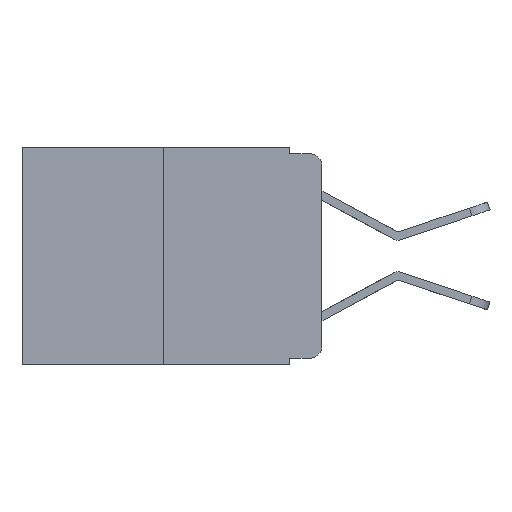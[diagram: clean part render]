
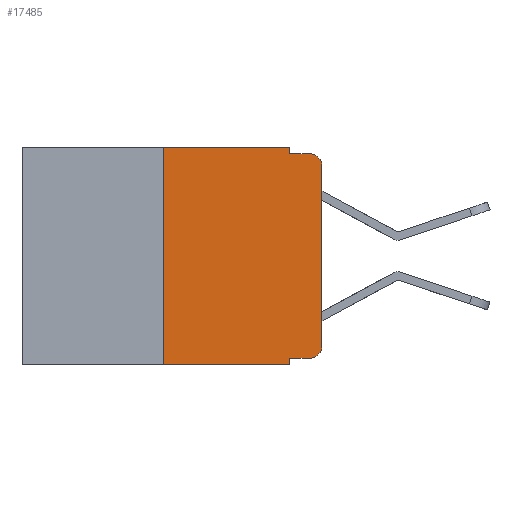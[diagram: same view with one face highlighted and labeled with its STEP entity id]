
A CAD part, left-side view. The second image highlights one B-rep face of the part: STEP entity #17485.
In plain terms, the highlighted planar face has unit normal (-1, 0, 0).
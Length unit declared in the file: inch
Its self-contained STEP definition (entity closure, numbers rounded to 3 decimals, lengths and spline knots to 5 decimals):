
#33 = CARTESIAN_POINT ( 'NONE',  ( 0., 0., -0.03 ) ) ;
#258 = CARTESIAN_POINT ( 'NONE',  ( 0., 0.25, 0. ) ) ;
#469 = LINE ( 'NONE', #2972, #22133 ) ;
#549 = VERTEX_POINT ( 'NONE', #8076 ) ;
#557 = DIRECTION ( 'NONE',  ( 0., 0., -1. ) ) ;
#564 = CARTESIAN_POINT ( 'NONE',  ( 0., 0.051, -0.343 ) ) ;
#1714 = CARTESIAN_POINT ( 'NONE',  ( 0., 0.051, -0.01 ) ) ;
#1905 = VECTOR ( 'NONE', #4295, 39.37008 ) ;
#1937 = AXIS2_PLACEMENT_3D ( 'NONE', #16256, #14419, #10748 ) ;
#1993 = VECTOR ( 'NONE', #10493, 39.37008 ) ;
#2056 = ORIENTED_EDGE ( 'NONE', *, *, #19899, .T. ) ;
#2554 = AXIS2_PLACEMENT_3D ( 'NONE', #11910, #4063, #8116 ) ;
#2972 = CARTESIAN_POINT ( 'NONE',  ( 0., 0.051, -0.333 ) ) ;
#3276 = ORIENTED_EDGE ( 'NONE', *, *, #23657, .T. ) ;
#3572 = CIRCLE ( 'NONE', #2554, 0.02 ) ;
#3613 = VERTEX_POINT ( 'NONE', #564 ) ;
#3642 = DIRECTION ( 'NONE',  ( 0., -1., 0. ) ) ;
#3661 = VERTEX_POINT ( 'NONE', #4584 ) ;
#3707 = LINE ( 'NONE', #8032, #1905 ) ;
#3794 = DIRECTION ( 'NONE',  ( 0., -1., 0. ) ) ;
#4063 = DIRECTION ( 'NONE',  ( -1., 0., 0. ) ) ;
#4295 = DIRECTION ( 'NONE',  ( 0., 0., 1. ) ) ;
#4326 = VERTEX_POINT ( 'NONE', #21395 ) ;
#4584 = CARTESIAN_POINT ( 'NONE',  ( 0., 0.25, -0.343 ) ) ;
#4634 = DIRECTION ( 'NONE',  ( 0., -1., 0. ) ) ;
#4813 = EDGE_CURVE ( 'NONE', #3661, #18534, #3707, .T. ) ;
#5150 = EDGE_CURVE ( 'NONE', #18534, #549, #18207, .T. ) ;
#6787 = CARTESIAN_POINT ( 'NONE',  ( 0., 0.051, 0. ) ) ;
#7406 = VERTEX_POINT ( 'NONE', #22381 ) ;
#7524 = VERTEX_POINT ( 'NONE', #33 ) ;
#8032 = CARTESIAN_POINT ( 'NONE',  ( 0., 0.25, 0. ) ) ;
#8076 = CARTESIAN_POINT ( 'NONE',  ( 0., 0.051, 0. ) ) ;
#8116 = DIRECTION ( 'NONE',  ( 0., 0., -1. ) ) ;
#8274 = EDGE_CURVE ( 'NONE', #8920, #7406, #10379, .T. ) ;
#8920 = VERTEX_POINT ( 'NONE', #23215 ) ;
#9047 = VECTOR ( 'NONE', #14927, 39.37008 ) ;
#9711 = LINE ( 'NONE', #6787, #18607 ) ;
#9781 = ORIENTED_EDGE ( 'NONE', *, *, #4813, .F. ) ;
#9878 = FACE_OUTER_BOUND ( 'NONE', #10364, .T. ) ;
#10024 = PLANE ( 'NONE',  #17247 ) ;
#10364 = EDGE_LOOP ( 'NONE', ( #14322, #15340, #22696, #15757, #14971, #9781, #19636, #17061, #2056, #3276 ) ) ;
#10379 = LINE ( 'NONE', #1714, #12759 ) ;
#10493 = DIRECTION ( 'NONE',  ( 0., 0., -1. ) ) ;
#10511 = DIRECTION ( 'NONE',  ( 0., 0., 1. ) ) ;
#10748 = DIRECTION ( 'NONE',  ( 0., 0., -1. ) ) ;
#11910 = CARTESIAN_POINT ( 'NONE',  ( 0., 0.02, -0.313 ) ) ;
#11927 = DIRECTION ( 'NONE',  ( 1., 0., 0. ) ) ;
#11982 = LINE ( 'NONE', #18602, #9047 ) ;
#12033 = EDGE_CURVE ( 'NONE', #7524, #7406, #23340, .T. ) ;
#12048 = EDGE_CURVE ( 'NONE', #549, #8920, #9711, .T. ) ;
#12759 = VECTOR ( 'NONE', #3642, 39.37008 ) ;
#13300 = VECTOR ( 'NONE', #10511, 39.37008 ) ;
#14263 = CARTESIAN_POINT ( 'NONE',  ( 0., 0.051, 0. ) ) ;
#14322 = ORIENTED_EDGE ( 'NONE', *, *, #23898, .T. ) ;
#14419 = DIRECTION ( 'NONE',  ( -1., 0., 0. ) ) ;
#14667 = DIRECTION ( 'NONE',  ( 0., 0., -1. ) ) ;
#14927 = DIRECTION ( 'NONE',  ( 0., -1., 0. ) ) ;
#14971 = ORIENTED_EDGE ( 'NONE', *, *, #5150, .F. ) ;
#15340 = ORIENTED_EDGE ( 'NONE', *, *, #12033, .T. ) ;
#15757 = ORIENTED_EDGE ( 'NONE', *, *, #12048, .F. ) ;
#16256 = CARTESIAN_POINT ( 'NONE',  ( 0., 0.02, -0.03 ) ) ;
#16284 = CARTESIAN_POINT ( 'NONE',  ( 0., 0., 0. ) ) ;
#16667 = EDGE_CURVE ( 'NONE', #3661, #3613, #11982, .T. ) ;
#17061 = ORIENTED_EDGE ( 'NONE', *, *, #19862, .F. ) ;
#17247 = AXIS2_PLACEMENT_3D ( 'NONE', #19617, #11927, #557 ) ;
#17485 = ADVANCED_FACE ( 'NONE', ( #9878 ), #10024, .F. ) ;
#17738 = CARTESIAN_POINT ( 'NONE',  ( 0., 0.051, -0.333 ) ) ;
#17998 = LINE ( 'NONE', #14263, #1993 ) ;
#18207 = LINE ( 'NONE', #20766, #23472 ) ;
#18374 = CARTESIAN_POINT ( 'NONE',  ( 0., 0.02, -0.333 ) ) ;
#18534 = VERTEX_POINT ( 'NONE', #258 ) ;
#18602 = CARTESIAN_POINT ( 'NONE',  ( 0., 0.473, -0.343 ) ) ;
#18607 = VECTOR ( 'NONE', #14667, 39.37008 ) ;
#19617 = CARTESIAN_POINT ( 'NONE',  ( 0., 0.473, 0. ) ) ;
#19636 = ORIENTED_EDGE ( 'NONE', *, *, #16667, .T. ) ;
#19862 = EDGE_CURVE ( 'NONE', #23109, #3613, #17998, .T. ) ;
#19899 = EDGE_CURVE ( 'NONE', #23109, #22171, #469, .T. ) ;
#20766 = CARTESIAN_POINT ( 'NONE',  ( 0., 0.473, 0. ) ) ;
#21395 = CARTESIAN_POINT ( 'NONE',  ( 0., 0., -0.313 ) ) ;
#22133 = VECTOR ( 'NONE', #4634, 39.37008 ) ;
#22171 = VERTEX_POINT ( 'NONE', #18374 ) ;
#22381 = CARTESIAN_POINT ( 'NONE',  ( 0., 0.02, -0.01 ) ) ;
#22696 = ORIENTED_EDGE ( 'NONE', *, *, #8274, .F. ) ;
#23109 = VERTEX_POINT ( 'NONE', #17738 ) ;
#23215 = CARTESIAN_POINT ( 'NONE',  ( 0., 0.051, -0.01 ) ) ;
#23340 = CIRCLE ( 'NONE', #1937, 0.02 ) ;
#23472 = VECTOR ( 'NONE', #3794, 39.37008 ) ;
#23657 = EDGE_CURVE ( 'NONE', #22171, #4326, #3572, .T. ) ;
#23898 = EDGE_CURVE ( 'NONE', #4326, #7524, #23963, .T. ) ;
#23963 = LINE ( 'NONE', #16284, #13300 ) ;
